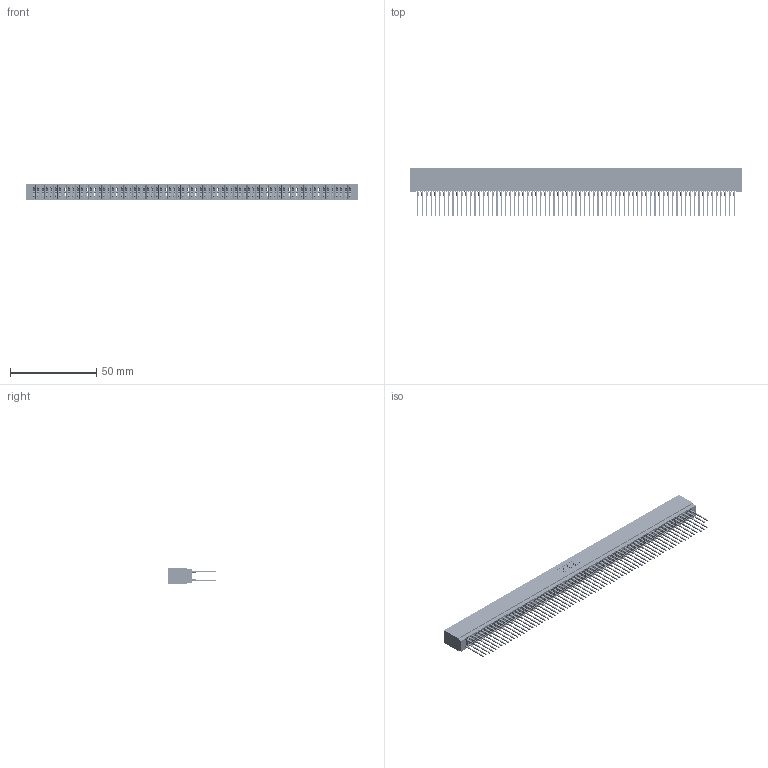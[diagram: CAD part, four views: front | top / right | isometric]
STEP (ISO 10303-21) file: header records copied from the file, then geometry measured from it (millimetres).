
FILE_DESCRIPTION (( 'STEP AP203' ), '1' );
FILE_NAME ('725-146-545-201.STEP', '2020-09-10T12:52:34', ( '' ), ( '' ), 'SwSTEP 2.0', 'SolidWorks 2020', '' );
FILE_SCHEMA (( 'CONFIG_CONTROL_DESIGN' ));
Products named in the file (3): 725 Part_Insulator Option - 01; 745-292-001_545; 725-146-545-201
Assembly tree (147 placements, depth 2):
  725-146-545-201
    725 Part_Insulator Option - 01
    745-292-001_545  x146
Bounding box: 192.02 x 28.21 x 8.89 mm (x, y, z)
Volume: 15584.7 mm3; surface area: 35810 mm2
Topology: 147 solids, 147 shells, 13162 faces, 35367 edges, 22214 vertices
Faces by surface type: plane 6771, bspline 2920, cylinder 2595, torus 876
Entity records: 118635 total; most frequent: CARTESIAN_POINT 21067, ORIENTED_EDGE 20564, DIRECTION 17940, EDGE_CURVE 10282, VECTOR 9662, LINE 9662, VERTEX_POINT 6554, AXIS2_PLACEMENT_3D 4139
